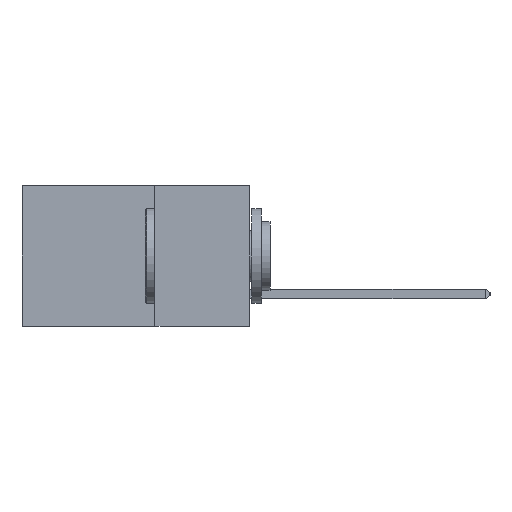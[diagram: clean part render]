
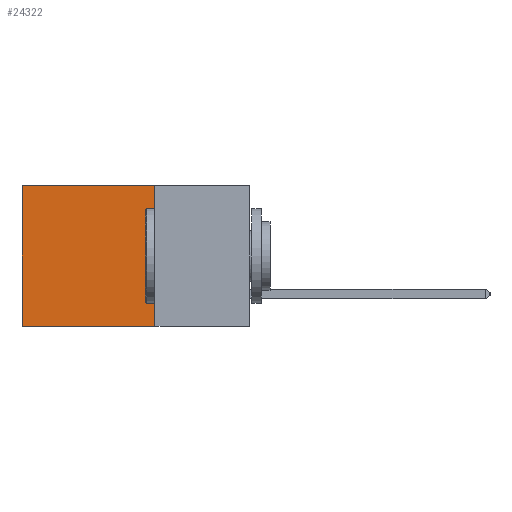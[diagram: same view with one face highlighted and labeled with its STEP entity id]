
A CAD part, left-side view. The second image highlights one B-rep face of the part: STEP entity #24322.
In plain terms, the highlighted planar face has unit normal (-1, 0, 0).
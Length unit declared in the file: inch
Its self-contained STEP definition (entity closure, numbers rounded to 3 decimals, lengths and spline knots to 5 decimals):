
#180 = AXIS2_PLACEMENT_3D ( 'NONE', #9469, #22709, #11395 ) ;
#791 = CARTESIAN_POINT ( 'NONE',  ( 0.2875, 0.6, 0. ) ) ;
#3040 = VECTOR ( 'NONE', #19352, 39.37008 ) ;
#3668 = LINE ( 'NONE', #17427, #3040 ) ;
#4231 = LINE ( 'NONE', #15613, #18952 ) ;
#5618 = EDGE_CURVE ( 'NONE', #22652, #10785, #21833, .T. ) ;
#5757 = ORIENTED_EDGE ( 'NONE', *, *, #20519, .T. ) ;
#5884 = DIRECTION ( 'NONE',  ( 0., 1., 0. ) ) ;
#5931 = FACE_OUTER_BOUND ( 'NONE', #19494, .T. ) ;
#6206 = ORIENTED_EDGE ( 'NONE', *, *, #13774, .T. ) ;
#6244 = VECTOR ( 'NONE', #21991, 39.37008 ) ;
#8714 = CARTESIAN_POINT ( 'NONE',  ( 0.2875, 0.25, 0. ) ) ;
#8730 = ORIENTED_EDGE ( 'NONE', *, *, #5618, .F. ) ;
#9469 = CARTESIAN_POINT ( 'NONE',  ( 0.2875, 0.25, 0. ) ) ;
#10785 = VERTEX_POINT ( 'NONE', #19177 ) ;
#11395 = DIRECTION ( 'NONE',  ( 0., 0., -1. ) ) ;
#12675 = CARTESIAN_POINT ( 'NONE',  ( 0.2875, 0.25, 0. ) ) ;
#13774 = EDGE_CURVE ( 'NONE', #20097, #10785, #3668, .T. ) ;
#15613 = CARTESIAN_POINT ( 'NONE',  ( 0.2875, 0.25, 0. ) ) ;
#16801 = VECTOR ( 'NONE', #5884, 39.37008 ) ;
#17267 = CARTESIAN_POINT ( 'NONE',  ( 0.2875, 0.25, -0.37 ) ) ;
#17427 = CARTESIAN_POINT ( 'NONE',  ( 0.2875, 0.6, 0. ) ) ;
#17514 = DIRECTION ( 'NONE',  ( 0., 1., 0. ) ) ;
#17933 = VERTEX_POINT ( 'NONE', #12675 ) ;
#18952 = VECTOR ( 'NONE', #17514, 39.37008 ) ;
#19177 = CARTESIAN_POINT ( 'NONE',  ( 0.2875, 0.6, -0.37 ) ) ;
#19352 = DIRECTION ( 'NONE',  ( 0., 0., -1. ) ) ;
#19494 = EDGE_LOOP ( 'NONE', ( #6206, #8730, #24519, #5757 ) ) ;
#20097 = VERTEX_POINT ( 'NONE', #791 ) ;
#20519 = EDGE_CURVE ( 'NONE', #17933, #20097, #4231, .T. ) ;
#20827 = PLANE ( 'NONE',  #180 ) ;
#21477 = LINE ( 'NONE', #8714, #6244 ) ;
#21833 = LINE ( 'NONE', #17267, #16801 ) ;
#21991 = DIRECTION ( 'NONE',  ( 0., 0., -1. ) ) ;
#22652 = VERTEX_POINT ( 'NONE', #23356 ) ;
#22709 = DIRECTION ( 'NONE',  ( 1., 0., 0. ) ) ;
#23356 = CARTESIAN_POINT ( 'NONE',  ( 0.2875, 0.25, -0.37 ) ) ;
#24083 = EDGE_CURVE ( 'NONE', #17933, #22652, #21477, .T. ) ;
#24322 = ADVANCED_FACE ( 'NONE', ( #5931 ), #20827, .F. ) ;
#24519 = ORIENTED_EDGE ( 'NONE', *, *, #24083, .F. ) ;
